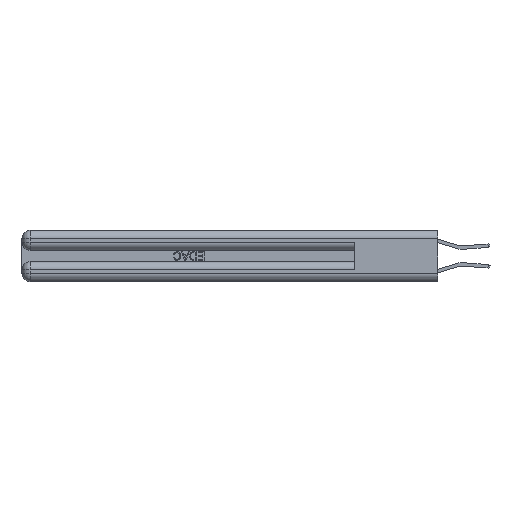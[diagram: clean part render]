
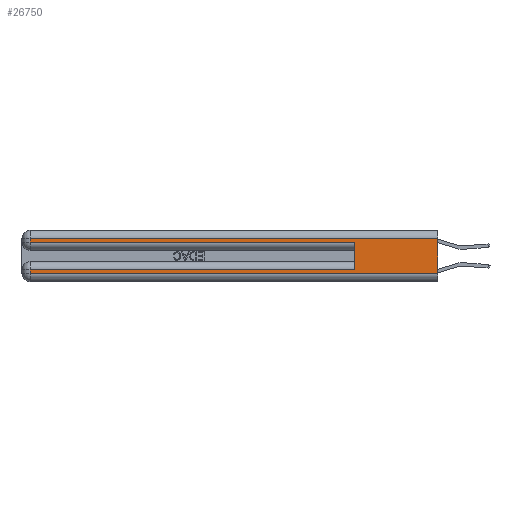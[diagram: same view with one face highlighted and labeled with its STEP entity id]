
A CAD part, left-side view. The second image highlights one B-rep face of the part: STEP entity #26750.
In plain terms, the highlighted planar face has unit normal (-1, 0, 0).
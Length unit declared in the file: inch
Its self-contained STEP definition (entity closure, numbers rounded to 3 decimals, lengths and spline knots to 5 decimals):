
#6 = EDGE_CURVE ( 'NONE', #82, #24985, #24448, .T. ) ;
#82 = VERTEX_POINT ( 'NONE', #19852 ) ;
#446 = EDGE_LOOP ( 'NONE', ( #10090, #36218, #3067, #18784, #29316, #30383, #5115, #5885 ) ) ;
#692 = DIRECTION ( 'NONE',  ( 0., 0., -1. ) ) ;
#1402 = CARTESIAN_POINT ( 'NONE',  ( 0., 0., 0.085 ) ) ;
#1604 = VECTOR ( 'NONE', #4710, 39.37008 ) ;
#2081 = CARTESIAN_POINT ( 'NONE',  ( 0., 2.94, 0.31 ) ) ;
#2112 = LINE ( 'NONE', #2303, #17496 ) ;
#2303 = CARTESIAN_POINT ( 'NONE',  ( 0., 0., 0.31 ) ) ;
#3067 = ORIENTED_EDGE ( 'NONE', *, *, #30211, .T. ) ;
#4710 = DIRECTION ( 'NONE',  ( 0., 0., -1. ) ) ;
#4792 = VERTEX_POINT ( 'NONE', #13385 ) ;
#5115 = ORIENTED_EDGE ( 'NONE', *, *, #35510, .T. ) ;
#5317 = DIRECTION ( 'NONE',  ( 0., -1., 0. ) ) ;
#5448 = LINE ( 'NONE', #29200, #19902 ) ;
#5575 = CARTESIAN_POINT ( 'NONE',  ( 0., 0.6, 0.145 ) ) ;
#5885 = ORIENTED_EDGE ( 'NONE', *, *, #21478, .T. ) ;
#5900 = CARTESIAN_POINT ( 'NONE',  ( 0., 0., 0.06 ) ) ;
#6763 = CARTESIAN_POINT ( 'NONE',  ( 0., 2.94, 0.085 ) ) ;
#8300 = DIRECTION ( 'NONE',  ( 0., 1., 0. ) ) ;
#8598 = VECTOR ( 'NONE', #21542, 39.37008 ) ;
#9355 = CARTESIAN_POINT ( 'NONE',  ( 0., 0.6, 0.085 ) ) ;
#10090 = ORIENTED_EDGE ( 'NONE', *, *, #11589, .F. ) ;
#10420 = AXIS2_PLACEMENT_3D ( 'NONE', #12878, #18530, #35485 ) ;
#10851 = CARTESIAN_POINT ( 'NONE',  ( 0., 2.94, 0.37 ) ) ;
#11183 = FACE_OUTER_BOUND ( 'NONE', #446, .T. ) ;
#11559 = VECTOR ( 'NONE', #23509, 39.37008 ) ;
#11589 = EDGE_CURVE ( 'NONE', #16911, #17057, #5448, .T. ) ;
#11901 = EDGE_CURVE ( 'NONE', #22878, #24985, #33529, .T. ) ;
#12160 = EDGE_CURVE ( 'NONE', #22878, #27330, #30032, .T. ) ;
#12878 = CARTESIAN_POINT ( 'NONE',  ( 0., 0., 0.37 ) ) ;
#13385 = CARTESIAN_POINT ( 'NONE',  ( 0., 2.94, 0.06 ) ) ;
#13695 = DIRECTION ( 'NONE',  ( 0., 0., 1. ) ) ;
#14900 = VERTEX_POINT ( 'NONE', #2081 ) ;
#15241 = PLANE ( 'NONE',  #10420 ) ;
#16824 = VECTOR ( 'NONE', #5317, 39.37008 ) ;
#16839 = CARTESIAN_POINT ( 'NONE',  ( 0., 0., 0.06 ) ) ;
#16911 = VERTEX_POINT ( 'NONE', #26299 ) ;
#17057 = VERTEX_POINT ( 'NONE', #5900 ) ;
#17496 = VECTOR ( 'NONE', #8300, 39.37008 ) ;
#18530 = DIRECTION ( 'NONE',  ( 1., 0., 0. ) ) ;
#18784 = ORIENTED_EDGE ( 'NONE', *, *, #6, .T. ) ;
#19852 = CARTESIAN_POINT ( 'NONE',  ( 0., 2.94, 0.285 ) ) ;
#19902 = VECTOR ( 'NONE', #692, 39.37008 ) ;
#21478 = EDGE_CURVE ( 'NONE', #4792, #17057, #26964, .T. ) ;
#21542 = DIRECTION ( 'NONE',  ( 0., -1., 0. ) ) ;
#22878 = VERTEX_POINT ( 'NONE', #9355 ) ;
#23509 = DIRECTION ( 'NONE',  ( 0., 1., 0. ) ) ;
#24027 = LINE ( 'NONE', #10851, #1604 ) ;
#24326 = VECTOR ( 'NONE', #13695, 39.37008 ) ;
#24448 = LINE ( 'NONE', #32700, #8598 ) ;
#24560 = EDGE_CURVE ( 'NONE', #16911, #14900, #2112, .T. ) ;
#24985 = VERTEX_POINT ( 'NONE', #33809 ) ;
#26299 = CARTESIAN_POINT ( 'NONE',  ( 0., 0., 0.31 ) ) ;
#26750 = ADVANCED_FACE ( 'NONE', ( #11183 ), #15241, .F. ) ;
#26964 = LINE ( 'NONE', #16839, #16824 ) ;
#27330 = VERTEX_POINT ( 'NONE', #6763 ) ;
#28158 = VECTOR ( 'NONE', #34978, 39.37008 ) ;
#28585 = LINE ( 'NONE', #35249, #28158 ) ;
#29200 = CARTESIAN_POINT ( 'NONE',  ( 0., 0., 0.37 ) ) ;
#29316 = ORIENTED_EDGE ( 'NONE', *, *, #11901, .F. ) ;
#30032 = LINE ( 'NONE', #1402, #11559 ) ;
#30211 = EDGE_CURVE ( 'NONE', #14900, #82, #24027, .T. ) ;
#30383 = ORIENTED_EDGE ( 'NONE', *, *, #12160, .T. ) ;
#32700 = CARTESIAN_POINT ( 'NONE',  ( 0., 0., 0.285 ) ) ;
#33529 = LINE ( 'NONE', #5575, #24326 ) ;
#33809 = CARTESIAN_POINT ( 'NONE',  ( 0., 0.6, 0.285 ) ) ;
#34978 = DIRECTION ( 'NONE',  ( 0., 0., -1. ) ) ;
#35249 = CARTESIAN_POINT ( 'NONE',  ( 0., 2.94, 0.37 ) ) ;
#35485 = DIRECTION ( 'NONE',  ( 0., 0., -1. ) ) ;
#35510 = EDGE_CURVE ( 'NONE', #27330, #4792, #28585, .T. ) ;
#36218 = ORIENTED_EDGE ( 'NONE', *, *, #24560, .T. ) ;
